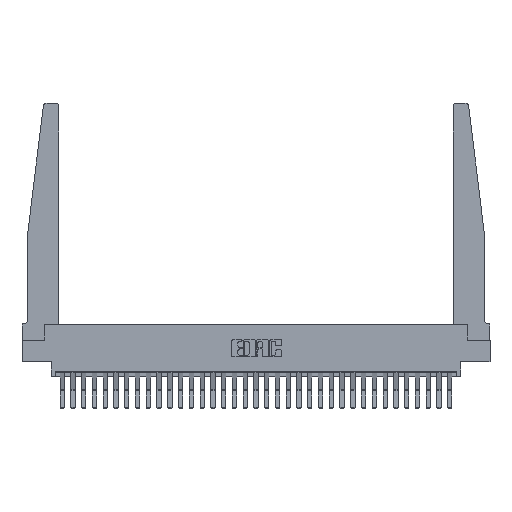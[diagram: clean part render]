
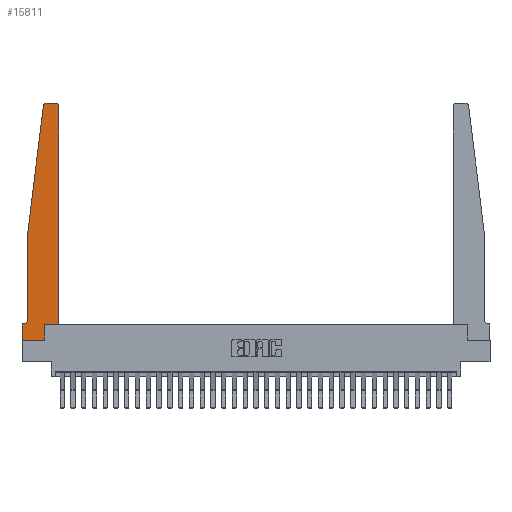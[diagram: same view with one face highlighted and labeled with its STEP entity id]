
A CAD part, top view. The second image highlights one B-rep face of the part: STEP entity #15811.
In plain terms, the highlighted planar face has unit normal (0, 0, 1).
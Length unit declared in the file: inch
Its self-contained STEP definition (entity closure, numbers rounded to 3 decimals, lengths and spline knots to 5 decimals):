
#400 = AXIS2_PLACEMENT_3D ( 'NONE', #26162, #12328, #28503 ) ;
#444 = EDGE_CURVE ( 'NONE', #21704, #10029, #23435, .T. ) ;
#759 = CARTESIAN_POINT ( 'NONE',  ( 0., 0., 0.37 ) ) ;
#871 = EDGE_CURVE ( 'NONE', #8685, #13155, #6400, .T. ) ;
#1122 = ORIENTED_EDGE ( 'NONE', *, *, #22486, .T. ) ;
#1809 = CARTESIAN_POINT ( 'NONE',  ( 0.015, 0.1875, 0.37 ) ) ;
#1908 = LINE ( 'NONE', #24782, #24946 ) ;
#1928 = DIRECTION ( 'NONE',  ( 0., 1., 0. ) ) ;
#1929 = ORIENTED_EDGE ( 'NONE', *, *, #8813, .T. ) ;
#2102 = DIRECTION ( 'NONE',  ( -0.122, -0.992, 0. ) ) ;
#2883 = EDGE_CURVE ( 'NONE', #24878, #8421, #16389, .T. ) ;
#3410 = EDGE_CURVE ( 'NONE', #10830, #8685, #20362, .T. ) ;
#3764 = CARTESIAN_POINT ( 'NONE',  ( 0.395, 2.72, 0.37 ) ) ;
#3888 = VECTOR ( 'NONE', #24999, 39.37008 ) ;
#4403 = DIRECTION ( 'NONE',  ( 0., 0., -1. ) ) ;
#5140 = FACE_OUTER_BOUND ( 'NONE', #12088, .T. ) ;
#5261 = VECTOR ( 'NONE', #7001, 39.37008 ) ;
#5457 = AXIS2_PLACEMENT_3D ( 'NONE', #18219, #4403, #20564 ) ;
#5633 = AXIS2_PLACEMENT_3D ( 'NONE', #21027, #7201, #23368 ) ;
#6058 = DIRECTION ( 'NONE',  ( 1., 0., 0. ) ) ;
#6400 = LINE ( 'NONE', #19718, #12549 ) ;
#7001 = DIRECTION ( 'NONE',  ( 1., 0., 0. ) ) ;
#7049 = VERTEX_POINT ( 'NONE', #23904 ) ;
#7201 = DIRECTION ( 'NONE',  ( 0., 0., 1. ) ) ;
#7348 = ORIENTED_EDGE ( 'NONE', *, *, #14131, .T. ) ;
#8421 = VERTEX_POINT ( 'NONE', #16830 ) ;
#8685 = VERTEX_POINT ( 'NONE', #20064 ) ;
#8701 = CARTESIAN_POINT ( 'NONE',  ( 0.065, 0.1875, 0.37 ) ) ;
#8756 = CARTESIAN_POINT ( 'NONE',  ( 0.2605, 0.18, 0.37 ) ) ;
#8813 = EDGE_CURVE ( 'NONE', #23167, #19972, #22308, .T. ) ;
#9355 = LINE ( 'NONE', #13626, #15505 ) ;
#9757 = CARTESIAN_POINT ( 'NONE',  ( 0., 0.1875, 0.37 ) ) ;
#10017 = PLANE ( 'NONE',  #400 ) ;
#10029 = VERTEX_POINT ( 'NONE', #9757 ) ;
#10418 = DIRECTION ( 'NONE',  ( -1., 0., 0. ) ) ;
#10712 = ORIENTED_EDGE ( 'NONE', *, *, #871, .T. ) ;
#10830 = VERTEX_POINT ( 'NONE', #28828 ) ;
#10991 = CARTESIAN_POINT ( 'NONE',  ( 0.2605, 0.18, 0.37 ) ) ;
#11495 = CARTESIAN_POINT ( 'NONE',  ( 0.2605, 0., 0.37 ) ) ;
#11585 = DIRECTION ( 'NONE',  ( -1., 0., 0. ) ) ;
#12088 = EDGE_LOOP ( 'NONE', ( #10712, #28568, #16213, #22136, #1122, #29401, #18556, #7348, #1929, #25983, #28438, #25847 ) ) ;
#12328 = DIRECTION ( 'NONE',  ( 0., 0., 1. ) ) ;
#12549 = VECTOR ( 'NONE', #10418, 39.37008 ) ;
#13053 = DIRECTION ( 'NONE',  ( 0., -1., 0. ) ) ;
#13155 = VERTEX_POINT ( 'NONE', #19154 ) ;
#13626 = CARTESIAN_POINT ( 'NONE',  ( 0.065, 1.25, 0.37 ) ) ;
#14131 = EDGE_CURVE ( 'NONE', #24966, #23167, #24406, .T. ) ;
#15505 = VECTOR ( 'NONE', #2102, 39.37008 ) ;
#15564 = LINE ( 'NONE', #24584, #20262 ) ;
#15683 = VECTOR ( 'NONE', #13053, 39.37008 ) ;
#15811 = ADVANCED_FACE ( 'NONE', ( #5140 ), #10017, .T. ) ;
#16213 = ORIENTED_EDGE ( 'NONE', *, *, #20044, .T. ) ;
#16389 = LINE ( 'NONE', #26893, #15683 ) ;
#16830 = CARTESIAN_POINT ( 'NONE',  ( 0.065, 0.2375, 0.37 ) ) ;
#17368 = VECTOR ( 'NONE', #1928, 39.37008 ) ;
#18219 = CARTESIAN_POINT ( 'NONE',  ( 0.015, 0.2375, 0.37 ) ) ;
#18342 = CARTESIAN_POINT ( 'NONE',  ( 0.065, 1.25, 0.37 ) ) ;
#18556 = ORIENTED_EDGE ( 'NONE', *, *, #19179, .T. ) ;
#18980 = VERTEX_POINT ( 'NONE', #19540 ) ;
#19134 = EDGE_CURVE ( 'NONE', #19972, #7049, #15564, .T. ) ;
#19154 = CARTESIAN_POINT ( 'NONE',  ( 0.27653, 2.75, 0.37 ) ) ;
#19179 = EDGE_CURVE ( 'NONE', #10029, #24966, #1908, .T. ) ;
#19274 = EDGE_CURVE ( 'NONE', #7049, #10830, #22792, .T. ) ;
#19540 = CARTESIAN_POINT ( 'NONE',  ( 0.24675, 2.72367, 0.37 ) ) ;
#19718 = CARTESIAN_POINT ( 'NONE',  ( 0.25, 2.75, 0.37 ) ) ;
#19888 = DIRECTION ( 'NONE',  ( 0., 0., 1. ) ) ;
#19972 = VERTEX_POINT ( 'NONE', #10991 ) ;
#20044 = EDGE_CURVE ( 'NONE', #18980, #24878, #9355, .T. ) ;
#20064 = CARTESIAN_POINT ( 'NONE',  ( 0.395, 2.75, 0.37 ) ) ;
#20262 = VECTOR ( 'NONE', #29239, 39.37008 ) ;
#20362 = CIRCLE ( 'NONE', #25297, 0.03 ) ;
#20564 = DIRECTION ( 'NONE',  ( -1., 0., 0. ) ) ;
#21027 = CARTESIAN_POINT ( 'NONE',  ( 0.27653, 2.72, 0.37 ) ) ;
#21376 = EDGE_CURVE ( 'NONE', #13155, #18980, #24464, .T. ) ;
#21704 = VERTEX_POINT ( 'NONE', #1809 ) ;
#22136 = ORIENTED_EDGE ( 'NONE', *, *, #2883, .T. ) ;
#22308 = LINE ( 'NONE', #8756, #3888 ) ;
#22486 = EDGE_CURVE ( 'NONE', #8421, #21704, #22967, .T. ) ;
#22792 = LINE ( 'NONE', #25072, #17368 ) ;
#22967 = CIRCLE ( 'NONE', #5457, 0.05 ) ;
#23167 = VERTEX_POINT ( 'NONE', #11495 ) ;
#23368 = DIRECTION ( 'NONE',  ( 1., 0., 0. ) ) ;
#23435 = LINE ( 'NONE', #8701, #28857 ) ;
#23904 = CARTESIAN_POINT ( 'NONE',  ( 0.425, 0.18, 0.37 ) ) ;
#24406 = LINE ( 'NONE', #25369, #5261 ) ;
#24464 = CIRCLE ( 'NONE', #5633, 0.03 ) ;
#24584 = CARTESIAN_POINT ( 'NONE',  ( 0.425, 0.18, 0.37 ) ) ;
#24782 = CARTESIAN_POINT ( 'NONE',  ( 0., 0., 0.37 ) ) ;
#24878 = VERTEX_POINT ( 'NONE', #18342 ) ;
#24946 = VECTOR ( 'NONE', #27106, 39.37008 ) ;
#24966 = VERTEX_POINT ( 'NONE', #759 ) ;
#24999 = DIRECTION ( 'NONE',  ( 0., 1., 0. ) ) ;
#25072 = CARTESIAN_POINT ( 'NONE',  ( 0.425, 0.18, 0.37 ) ) ;
#25297 = AXIS2_PLACEMENT_3D ( 'NONE', #3764, #19888, #6058 ) ;
#25369 = CARTESIAN_POINT ( 'NONE',  ( 0., 0., 0.37 ) ) ;
#25847 = ORIENTED_EDGE ( 'NONE', *, *, #3410, .T. ) ;
#25983 = ORIENTED_EDGE ( 'NONE', *, *, #19134, .T. ) ;
#26162 = CARTESIAN_POINT ( 'NONE',  ( 0., 0.1875, 0.37 ) ) ;
#26893 = CARTESIAN_POINT ( 'NONE',  ( 0.065, 1.25, 0.37 ) ) ;
#27106 = DIRECTION ( 'NONE',  ( 0., -1., 0. ) ) ;
#28438 = ORIENTED_EDGE ( 'NONE', *, *, #19274, .T. ) ;
#28503 = DIRECTION ( 'NONE',  ( 1., 0., 0. ) ) ;
#28568 = ORIENTED_EDGE ( 'NONE', *, *, #21376, .T. ) ;
#28828 = CARTESIAN_POINT ( 'NONE',  ( 0.425, 2.72, 0.37 ) ) ;
#28857 = VECTOR ( 'NONE', #11585, 39.37008 ) ;
#29239 = DIRECTION ( 'NONE',  ( 1., 0., 0. ) ) ;
#29401 = ORIENTED_EDGE ( 'NONE', *, *, #444, .T. ) ;
